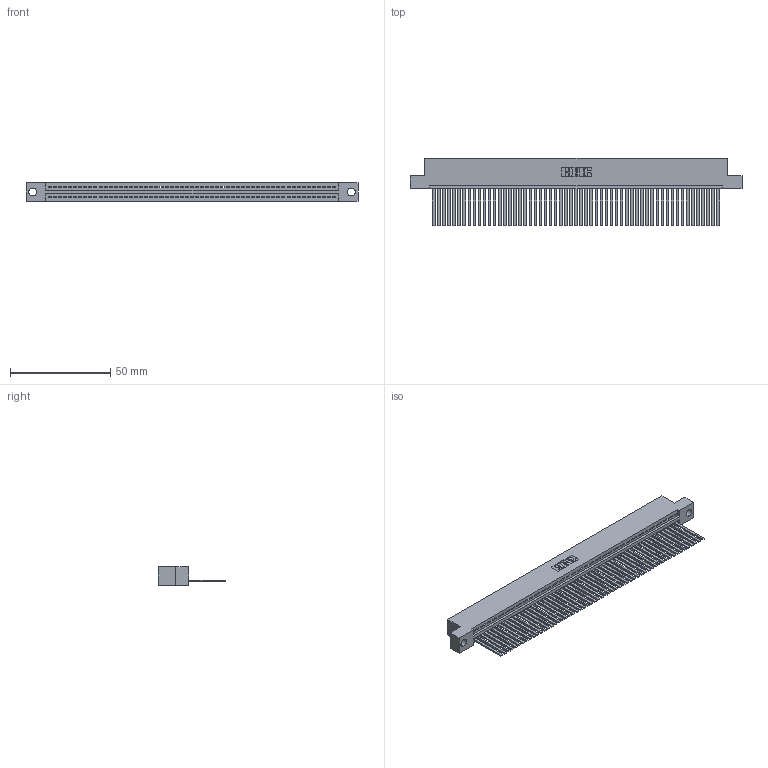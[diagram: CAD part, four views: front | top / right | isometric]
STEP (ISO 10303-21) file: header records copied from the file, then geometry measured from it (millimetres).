
FILE_DESCRIPTION (( 'STEP AP203' ), '1' );
FILE_NAME ('395-057-544-104.STEP', '2018-11-22T23:03:26', ( '' ), ( '' ), 'SwSTEP 2.0', 'SolidWorks 2016', '' );
FILE_SCHEMA (( 'CONFIG_CONTROL_DESIGN' ));
Length unit declared in the file: inch
Products named in the file (3): 345-292-001_345-293-144; 395-057-544-104; 345 Part_Flush Mounting Lugs - 0.156 Dia-TH
Assembly tree (58 placements, depth 2):
  395-057-544-104
    345 Part_Flush Mounting Lugs - 0.156 Dia-TH
    345-292-001_345-293-144  x57
Bounding box: 165.99 x 33.96 x 9.4 mm (x, y, z)
Volume: 16461 mm3; surface area: 23869.5 mm2
Topology: 58 solids, 58 shells, 3090 faces, 9347 edges, 6154 vertices
Faces by surface type: plane 2132, cylinder 958
Entity records: 40699 total; most frequent: CARTESIAN_POINT 7055, ORIENTED_EDGE 7046, DIRECTION 6137, EDGE_CURVE 3523, VECTOR 3167, LINE 3167, VERTEX_POINT 2346, AXIS2_PLACEMENT_3D 1485
